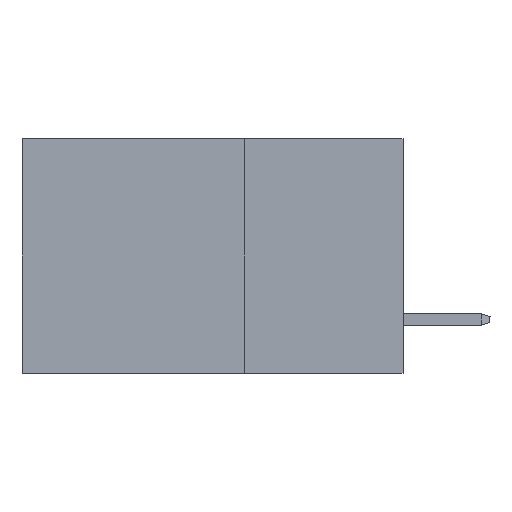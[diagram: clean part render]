
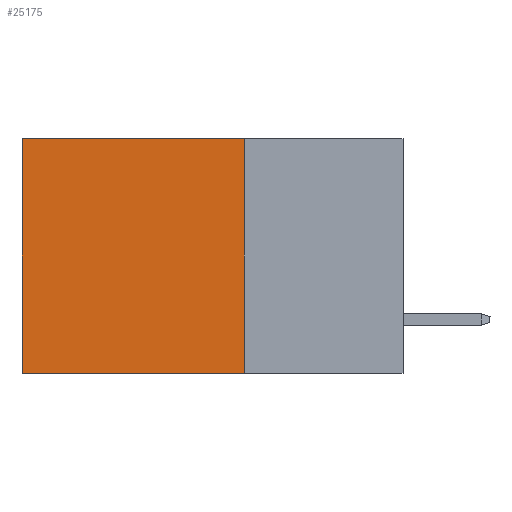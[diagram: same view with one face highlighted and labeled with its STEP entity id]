
A CAD part, left-side view. The second image highlights one B-rep face of the part: STEP entity #25175.
In plain terms, the highlighted planar face has unit normal (-1, 0, 0).
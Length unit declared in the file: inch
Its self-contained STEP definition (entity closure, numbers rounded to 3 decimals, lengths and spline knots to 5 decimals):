
#685 = EDGE_CURVE ( 'NONE', #23419, #7337, #28060, .T. ) ;
#2561 = ORIENTED_EDGE ( 'NONE', *, *, #6231, .T. ) ;
#2780 = DIRECTION ( 'NONE',  ( 0., 0., -1. ) ) ;
#3306 = EDGE_CURVE ( 'NONE', #23419, #20906, #9463, .T. ) ;
#3542 = CARTESIAN_POINT ( 'NONE',  ( 0.2875, 0.25, -0.37 ) ) ;
#4532 = LINE ( 'NONE', #14622, #16402 ) ;
#5894 = FACE_OUTER_BOUND ( 'NONE', #21972, .T. ) ;
#6231 = EDGE_CURVE ( 'NONE', #20906, #24671, #4532, .T. ) ;
#7337 = VERTEX_POINT ( 'NONE', #12746 ) ;
#7870 = DIRECTION ( 'NONE',  ( 0., 0., -1. ) ) ;
#9460 = AXIS2_PLACEMENT_3D ( 'NONE', #30558, #25489, #7870 ) ;
#9463 = LINE ( 'NONE', #11749, #19520 ) ;
#11749 = CARTESIAN_POINT ( 'NONE',  ( 0.2875, 0.25, 0. ) ) ;
#11975 = VECTOR ( 'NONE', #13634, 39.37008 ) ;
#12468 = CARTESIAN_POINT ( 'NONE',  ( 0.2875, 0.6, -0.37 ) ) ;
#12656 = CARTESIAN_POINT ( 'NONE',  ( 0.2875, 0.25, 0. ) ) ;
#12746 = CARTESIAN_POINT ( 'NONE',  ( 0.2875, 0.25, -0.37 ) ) ;
#13634 = DIRECTION ( 'NONE',  ( 0., 1., 0. ) ) ;
#13765 = ORIENTED_EDGE ( 'NONE', *, *, #685, .F. ) ;
#14622 = CARTESIAN_POINT ( 'NONE',  ( 0.2875, 0.6, 0. ) ) ;
#16402 = VECTOR ( 'NONE', #19038, 39.37008 ) ;
#16543 = EDGE_CURVE ( 'NONE', #7337, #24671, #28658, .T. ) ;
#19038 = DIRECTION ( 'NONE',  ( 0., 0., -1. ) ) ;
#19520 = VECTOR ( 'NONE', #22018, 39.37008 ) ;
#20904 = PLANE ( 'NONE',  #9460 ) ;
#20906 = VERTEX_POINT ( 'NONE', #31083 ) ;
#21912 = ORIENTED_EDGE ( 'NONE', *, *, #3306, .T. ) ;
#21972 = EDGE_LOOP ( 'NONE', ( #2561, #22021, #13765, #21912 ) ) ;
#22018 = DIRECTION ( 'NONE',  ( 0., 1., 0. ) ) ;
#22021 = ORIENTED_EDGE ( 'NONE', *, *, #16543, .F. ) ;
#23419 = VERTEX_POINT ( 'NONE', #12656 ) ;
#24277 = VECTOR ( 'NONE', #2780, 39.37008 ) ;
#24671 = VERTEX_POINT ( 'NONE', #12468 ) ;
#25175 = ADVANCED_FACE ( 'NONE', ( #5894 ), #20904, .F. ) ;
#25489 = DIRECTION ( 'NONE',  ( 1., 0., 0. ) ) ;
#28060 = LINE ( 'NONE', #28224, #24277 ) ;
#28224 = CARTESIAN_POINT ( 'NONE',  ( 0.2875, 0.25, 0. ) ) ;
#28658 = LINE ( 'NONE', #3542, #11975 ) ;
#30558 = CARTESIAN_POINT ( 'NONE',  ( 0.2875, 0.25, 0. ) ) ;
#31083 = CARTESIAN_POINT ( 'NONE',  ( 0.2875, 0.6, 0. ) ) ;
